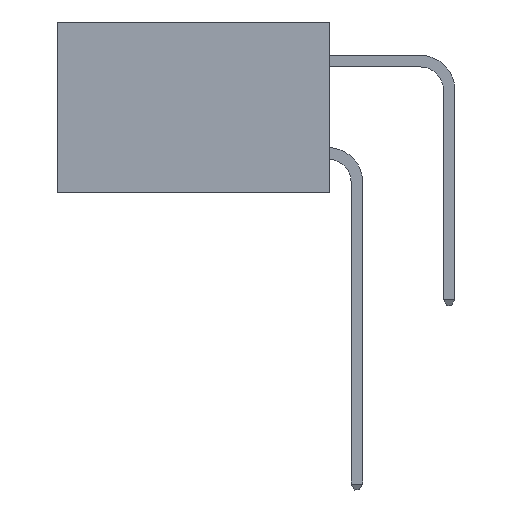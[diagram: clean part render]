
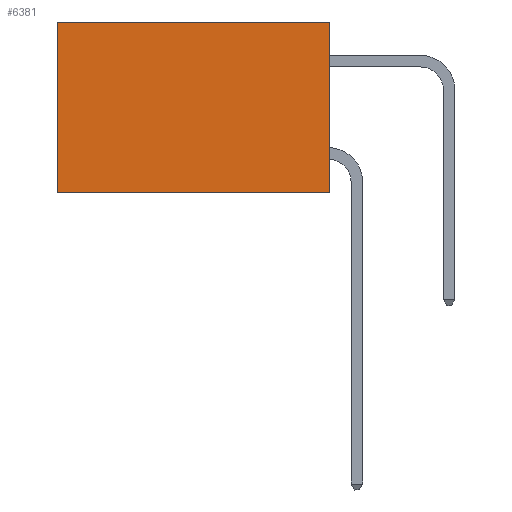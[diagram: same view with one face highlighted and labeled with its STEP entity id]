
A CAD part, left-side view. The second image highlights one B-rep face of the part: STEP entity #6381.
In plain terms, the highlighted planar face has unit normal (-1, 0, 0).
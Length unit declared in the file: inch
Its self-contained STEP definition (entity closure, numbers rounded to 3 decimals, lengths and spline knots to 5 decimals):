
#2207 = EDGE_CURVE ( 'NONE', #2963, #14830, #15505, .T. ) ;
#2548 = ORIENTED_EDGE ( 'NONE', *, *, #2207, .T. ) ;
#2738 = CARTESIAN_POINT ( 'NONE',  ( 0.277, 0., -0.37 ) ) ;
#2963 = VERTEX_POINT ( 'NONE', #9705 ) ;
#3553 = DIRECTION ( 'NONE',  ( 0., 0., -1. ) ) ;
#3689 = DIRECTION ( 'NONE',  ( 0., 0., -1. ) ) ;
#5058 = EDGE_LOOP ( 'NONE', ( #7512, #8697, #7733, #2548 ) ) ;
#5139 = EDGE_CURVE ( 'NONE', #11167, #7249, #9470, .T. ) ;
#5303 = EDGE_CURVE ( 'NONE', #2963, #11167, #12950, .T. ) ;
#5480 = CARTESIAN_POINT ( 'NONE',  ( 0.277, 0.59, 0. ) ) ;
#6381 = ADVANCED_FACE ( 'NONE', ( #15430 ), #14591, .F. ) ;
#6564 = VECTOR ( 'NONE', #3553, 39.37008 ) ;
#6835 = VECTOR ( 'NONE', #3689, 39.37008 ) ;
#6949 = LINE ( 'NONE', #14967, #6564 ) ;
#7147 = CARTESIAN_POINT ( 'NONE',  ( 0.277, 0., 0. ) ) ;
#7249 = VERTEX_POINT ( 'NONE', #14154 ) ;
#7386 = CARTESIAN_POINT ( 'NONE',  ( 0.277, 0., -0.37 ) ) ;
#7512 = ORIENTED_EDGE ( 'NONE', *, *, #7887, .T. ) ;
#7733 = ORIENTED_EDGE ( 'NONE', *, *, #5303, .F. ) ;
#7887 = EDGE_CURVE ( 'NONE', #14830, #7249, #6949, .T. ) ;
#8697 = ORIENTED_EDGE ( 'NONE', *, *, #5139, .F. ) ;
#8718 = VECTOR ( 'NONE', #11289, 39.37008 ) ;
#9470 = LINE ( 'NONE', #10913, #8718 ) ;
#9705 = CARTESIAN_POINT ( 'NONE',  ( 0.277, 0., 0. ) ) ;
#10913 = CARTESIAN_POINT ( 'NONE',  ( 0.277, 0., -0.37 ) ) ;
#11167 = VERTEX_POINT ( 'NONE', #2738 ) ;
#11289 = DIRECTION ( 'NONE',  ( 0., 1., 0. ) ) ;
#12295 = VECTOR ( 'NONE', #12868, 39.37008 ) ;
#12868 = DIRECTION ( 'NONE',  ( 0., 1., 0. ) ) ;
#12950 = LINE ( 'NONE', #7386, #6835 ) ;
#14154 = CARTESIAN_POINT ( 'NONE',  ( 0.277, 0.59, -0.37 ) ) ;
#14184 = AXIS2_PLACEMENT_3D ( 'NONE', #14335, #14604, #14685 ) ;
#14335 = CARTESIAN_POINT ( 'NONE',  ( 0.277, 0., -0.37 ) ) ;
#14591 = PLANE ( 'NONE',  #14184 ) ;
#14604 = DIRECTION ( 'NONE',  ( 1., 0., 0. ) ) ;
#14685 = DIRECTION ( 'NONE',  ( 0., 0., -1. ) ) ;
#14830 = VERTEX_POINT ( 'NONE', #5480 ) ;
#14967 = CARTESIAN_POINT ( 'NONE',  ( 0.277, 0.59, -0.37 ) ) ;
#15430 = FACE_OUTER_BOUND ( 'NONE', #5058, .T. ) ;
#15505 = LINE ( 'NONE', #7147, #12295 ) ;
